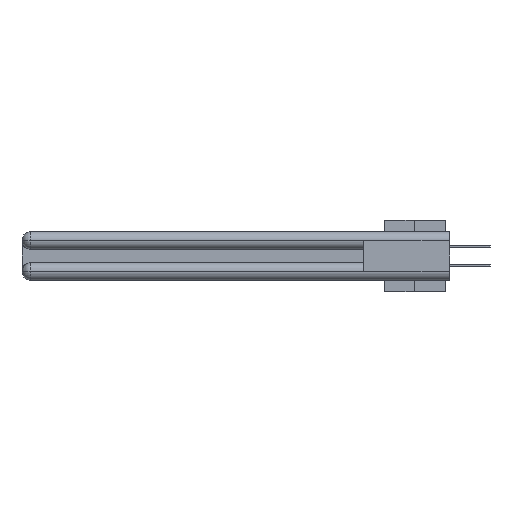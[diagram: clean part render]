
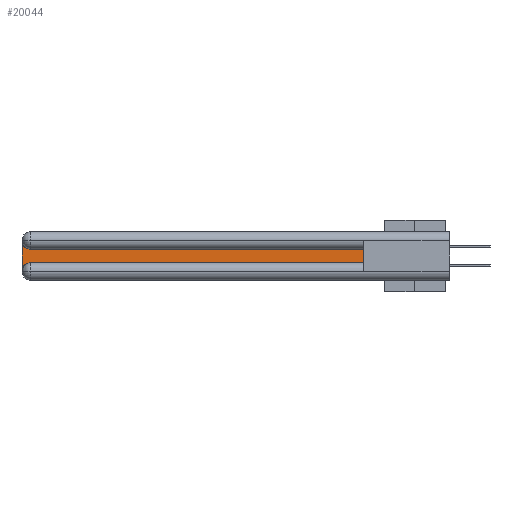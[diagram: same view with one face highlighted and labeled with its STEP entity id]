
A CAD part, left-side view. The second image highlights one B-rep face of the part: STEP entity #20044.
In plain terms, the highlighted planar face has unit normal (-1, 0, 0).
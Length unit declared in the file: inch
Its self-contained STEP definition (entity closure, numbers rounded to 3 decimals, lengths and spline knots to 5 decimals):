
#325 = DIRECTION ( 'NONE',  ( 0., 0., -1. ) ) ;
#366 = ORIENTED_EDGE ( 'NONE', *, *, #38569, .T. ) ;
#1434 = VERTEX_POINT ( 'NONE', #36151 ) ;
#2247 = EDGE_CURVE ( 'NONE', #14098, #9172, #38325, .T. ) ;
#2993 = DIRECTION ( 'NONE',  ( 0., 1., 0. ) ) ;
#3880 = CARTESIAN_POINT ( 'NONE',  ( 0.075, 2.94, -0.2175 ) ) ;
#4861 = VECTOR ( 'NONE', #2993, 39.37008 ) ;
#8977 = FACE_OUTER_BOUND ( 'NONE', #33755, .T. ) ;
#9172 = VERTEX_POINT ( 'NONE', #26441 ) ;
#9306 = CARTESIAN_POINT ( 'NONE',  ( 0.075, 3., -0.2175 ) ) ;
#9441 = CARTESIAN_POINT ( 'NONE',  ( 0.075, 0.6, -0.1225 ) ) ;
#10216 = CARTESIAN_POINT ( 'NONE',  ( 0.075, 0.6, -0.2175 ) ) ;
#10253 = VECTOR ( 'NONE', #28116, 39.37008 ) ;
#10343 = VERTEX_POINT ( 'NONE', #20186 ) ;
#12183 = LINE ( 'NONE', #9306, #10253 ) ;
#14098 = VERTEX_POINT ( 'NONE', #10216 ) ;
#14625 = EDGE_CURVE ( 'NONE', #1434, #19830, #12183, .T. ) ;
#14653 = EDGE_CURVE ( 'NONE', #9172, #10343, #16167, .T. ) ;
#15408 = AXIS2_PLACEMENT_3D ( 'NONE', #35691, #38662, #25987 ) ;
#15974 = VECTOR ( 'NONE', #19005, 39.37008 ) ;
#16167 = LINE ( 'NONE', #9441, #4861 ) ;
#16328 = CIRCLE ( 'NONE', #15408, 0.06 ) ;
#16457 = DIRECTION ( 'NONE',  ( 0., 0., 1. ) ) ;
#17218 = ORIENTED_EDGE ( 'NONE', *, *, #14625, .T. ) ;
#19005 = DIRECTION ( 'NONE',  ( 0., -1., 0. ) ) ;
#19061 = CARTESIAN_POINT ( 'NONE',  ( 0.075, 3., -0.2775 ) ) ;
#19830 = VERTEX_POINT ( 'NONE', #19061 ) ;
#20044 = ADVANCED_FACE ( 'NONE', ( #8977 ), #37230, .F. ) ;
#20186 = CARTESIAN_POINT ( 'NONE',  ( 0.075, 2.94, -0.1225 ) ) ;
#20213 = VERTEX_POINT ( 'NONE', #3880 ) ;
#21371 = AXIS2_PLACEMENT_3D ( 'NONE', #38176, #31626, #325 ) ;
#25987 = DIRECTION ( 'NONE',  ( 0., 0., -1. ) ) ;
#26105 = CARTESIAN_POINT ( 'NONE',  ( 0.075, 0.6, -0.2175 ) ) ;
#26211 = AXIS2_PLACEMENT_3D ( 'NONE', #37637, #31077, #28327 ) ;
#26441 = CARTESIAN_POINT ( 'NONE',  ( 0.075, 0.6, -0.1225 ) ) ;
#27404 = ORIENTED_EDGE ( 'NONE', *, *, #30009, .T. ) ;
#28116 = DIRECTION ( 'NONE',  ( 0., 0., -1. ) ) ;
#28229 = CARTESIAN_POINT ( 'NONE',  ( 0.075, 0.6, -0.2175 ) ) ;
#28327 = DIRECTION ( 'NONE',  ( 0., 0., -1. ) ) ;
#28351 = ORIENTED_EDGE ( 'NONE', *, *, #38757, .T. ) ;
#30009 = EDGE_CURVE ( 'NONE', #20213, #14098, #30107, .T. ) ;
#30031 = VECTOR ( 'NONE', #16457, 39.37008 ) ;
#30107 = LINE ( 'NONE', #28229, #15974 ) ;
#31077 = DIRECTION ( 'NONE',  ( 1., 0., 0. ) ) ;
#31626 = DIRECTION ( 'NONE',  ( 1., 0., 0. ) ) ;
#33318 = ORIENTED_EDGE ( 'NONE', *, *, #14653, .T. ) ;
#33755 = EDGE_LOOP ( 'NONE', ( #33318, #366, #17218, #28351, #27404, #34322 ) ) ;
#34322 = ORIENTED_EDGE ( 'NONE', *, *, #2247, .T. ) ;
#35691 = CARTESIAN_POINT ( 'NONE',  ( 0.075, 2.94, -0.0625 ) ) ;
#36151 = CARTESIAN_POINT ( 'NONE',  ( 0.075, 3., -0.0625 ) ) ;
#37230 = PLANE ( 'NONE',  #26211 ) ;
#37637 = CARTESIAN_POINT ( 'NONE',  ( 0.075, 3., -0.1225 ) ) ;
#38176 = CARTESIAN_POINT ( 'NONE',  ( 0.075, 2.94, -0.2775 ) ) ;
#38325 = LINE ( 'NONE', #26105, #30031 ) ;
#38569 = EDGE_CURVE ( 'NONE', #10343, #1434, #16328, .T. ) ;
#38662 = DIRECTION ( 'NONE',  ( 1., 0., 0. ) ) ;
#38757 = EDGE_CURVE ( 'NONE', #19830, #20213, #40171, .T. ) ;
#40171 = CIRCLE ( 'NONE', #21371, 0.06 ) ;
